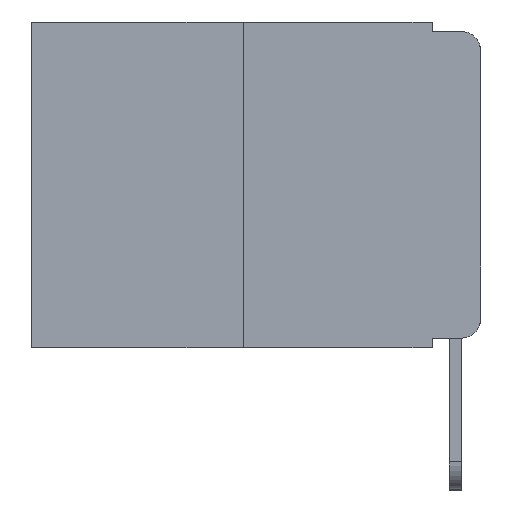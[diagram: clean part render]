
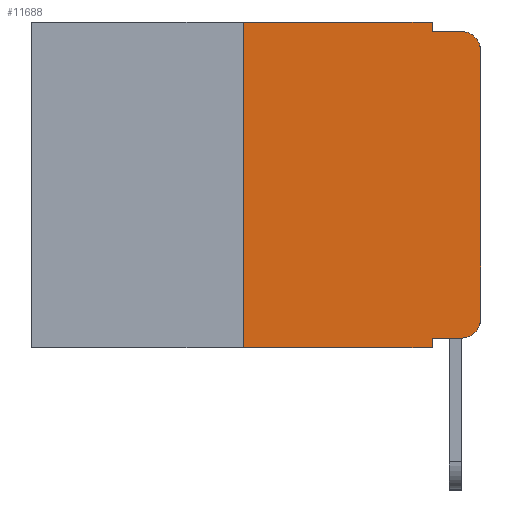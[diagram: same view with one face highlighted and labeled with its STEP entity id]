
A CAD part, left-side view. The second image highlights one B-rep face of the part: STEP entity #11688.
In plain terms, the highlighted planar face has unit normal (-1, 0, 0).
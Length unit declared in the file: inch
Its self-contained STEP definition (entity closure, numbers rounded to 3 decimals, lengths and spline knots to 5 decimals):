
#247 = DIRECTION ( 'NONE',  ( 0., 0., -1. ) ) ;
#393 = CARTESIAN_POINT ( 'NONE',  ( 0., 0.051, -0.333 ) ) ;
#453 = CARTESIAN_POINT ( 'NONE',  ( 0., 0., -0.313 ) ) ;
#469 = VECTOR ( 'NONE', #12345, 39.37008 ) ;
#862 = ORIENTED_EDGE ( 'NONE', *, *, #11897, .F. ) ;
#910 = DIRECTION ( 'NONE',  ( 0., -1., 0. ) ) ;
#989 = CARTESIAN_POINT ( 'NONE',  ( 0., 0.25, 0. ) ) ;
#1077 = DIRECTION ( 'NONE',  ( 0., 0., -1. ) ) ;
#1086 = EDGE_CURVE ( 'NONE', #10923, #11331, #10869, .T. ) ;
#1088 = DIRECTION ( 'NONE',  ( 0., -1., 0. ) ) ;
#1341 = EDGE_LOOP ( 'NONE', ( #8229, #8636, #10914, #2355, #1882, #6514, #6603, #862, #5809, #4588 ) ) ;
#1342 = DIRECTION ( 'NONE',  ( -1., 0., 0. ) ) ;
#1620 = VECTOR ( 'NONE', #12644, 39.37008 ) ;
#1882 = ORIENTED_EDGE ( 'NONE', *, *, #1086, .F. ) ;
#2343 = CARTESIAN_POINT ( 'NONE',  ( 0., 0.473, 0. ) ) ;
#2355 = ORIENTED_EDGE ( 'NONE', *, *, #12616, .F. ) ;
#2583 = VECTOR ( 'NONE', #9822, 39.37008 ) ;
#2612 = VERTEX_POINT ( 'NONE', #453 ) ;
#2708 = VERTEX_POINT ( 'NONE', #12746 ) ;
#2729 = VECTOR ( 'NONE', #10475, 39.37008 ) ;
#2891 = VECTOR ( 'NONE', #7727, 39.37008 ) ;
#2892 = CIRCLE ( 'NONE', #10574, 0.02 ) ;
#2956 = CARTESIAN_POINT ( 'NONE',  ( 0., 0., -0.03 ) ) ;
#3843 = CARTESIAN_POINT ( 'NONE',  ( 0., 0.051, 0. ) ) ;
#4492 = AXIS2_PLACEMENT_3D ( 'NONE', #7003, #6009, #12083 ) ;
#4588 = ORIENTED_EDGE ( 'NONE', *, *, #9158, .T. ) ;
#4644 = LINE ( 'NONE', #10712, #2891 ) ;
#4702 = LINE ( 'NONE', #7176, #11102 ) ;
#4929 = LINE ( 'NONE', #9195, #10697 ) ;
#5020 = CARTESIAN_POINT ( 'NONE',  ( 0., 0.051, -0.343 ) ) ;
#5229 = CARTESIAN_POINT ( 'NONE',  ( 0., 0., 0. ) ) ;
#5346 = CARTESIAN_POINT ( 'NONE',  ( 0., 0.25, 0. ) ) ;
#5636 = CARTESIAN_POINT ( 'NONE',  ( 0., 0.051, 0. ) ) ;
#5809 = ORIENTED_EDGE ( 'NONE', *, *, #6501, .T. ) ;
#6009 = DIRECTION ( 'NONE',  ( -1., 0., 0. ) ) ;
#6055 = LINE ( 'NONE', #393, #1620 ) ;
#6311 = CARTESIAN_POINT ( 'NONE',  ( 0., 0.051, -0.01 ) ) ;
#6501 = EDGE_CURVE ( 'NONE', #7918, #8531, #6055, .T. ) ;
#6514 = ORIENTED_EDGE ( 'NONE', *, *, #11779, .F. ) ;
#6603 = ORIENTED_EDGE ( 'NONE', *, *, #6868, .T. ) ;
#6658 = LINE ( 'NONE', #5636, #13190 ) ;
#6841 = EDGE_CURVE ( 'NONE', #10787, #2708, #12117, .T. ) ;
#6868 = EDGE_CURVE ( 'NONE', #13175, #12124, #4929, .T. ) ;
#7003 = CARTESIAN_POINT ( 'NONE',  ( 0., 0.02, -0.03 ) ) ;
#7176 = CARTESIAN_POINT ( 'NONE',  ( 0., 0.051, -0.01 ) ) ;
#7637 = VERTEX_POINT ( 'NONE', #6311 ) ;
#7662 = EDGE_CURVE ( 'NONE', #2612, #10787, #11311, .T. ) ;
#7727 = DIRECTION ( 'NONE',  ( 0., 0., -1. ) ) ;
#7918 = VERTEX_POINT ( 'NONE', #11704 ) ;
#8229 = ORIENTED_EDGE ( 'NONE', *, *, #7662, .T. ) ;
#8432 = CARTESIAN_POINT ( 'NONE',  ( 0., 0.02, -0.333 ) ) ;
#8531 = VERTEX_POINT ( 'NONE', #8432 ) ;
#8636 = ORIENTED_EDGE ( 'NONE', *, *, #6841, .T. ) ;
#9158 = EDGE_CURVE ( 'NONE', #8531, #2612, #2892, .T. ) ;
#9195 = CARTESIAN_POINT ( 'NONE',  ( 0., 0.473, -0.343 ) ) ;
#9479 = DIRECTION ( 'NONE',  ( 1., 0., 0. ) ) ;
#9592 = CARTESIAN_POINT ( 'NONE',  ( 0., 0.02, -0.313 ) ) ;
#9822 = DIRECTION ( 'NONE',  ( 0., 0., 1. ) ) ;
#10085 = AXIS2_PLACEMENT_3D ( 'NONE', #2343, #9479, #247 ) ;
#10475 = DIRECTION ( 'NONE',  ( 0., -1., 0. ) ) ;
#10574 = AXIS2_PLACEMENT_3D ( 'NONE', #9592, #1342, #12613 ) ;
#10608 = CARTESIAN_POINT ( 'NONE',  ( 0., 0.473, 0. ) ) ;
#10697 = VECTOR ( 'NONE', #910, 39.37008 ) ;
#10712 = CARTESIAN_POINT ( 'NONE',  ( 0., 0.051, 0. ) ) ;
#10787 = VERTEX_POINT ( 'NONE', #2956 ) ;
#10869 = LINE ( 'NONE', #10608, #2729 ) ;
#10914 = ORIENTED_EDGE ( 'NONE', *, *, #12159, .F. ) ;
#10923 = VERTEX_POINT ( 'NONE', #989 ) ;
#11102 = VECTOR ( 'NONE', #1088, 39.37008 ) ;
#11311 = LINE ( 'NONE', #5229, #469 ) ;
#11331 = VERTEX_POINT ( 'NONE', #3843 ) ;
#11688 = ADVANCED_FACE ( 'NONE', ( #12799 ), #12545, .F. ) ;
#11704 = CARTESIAN_POINT ( 'NONE',  ( 0., 0.051, -0.333 ) ) ;
#11779 = EDGE_CURVE ( 'NONE', #13175, #10923, #12951, .T. ) ;
#11897 = EDGE_CURVE ( 'NONE', #7918, #12124, #4644, .T. ) ;
#12083 = DIRECTION ( 'NONE',  ( 0., 0., -1. ) ) ;
#12117 = CIRCLE ( 'NONE', #4492, 0.02 ) ;
#12124 = VERTEX_POINT ( 'NONE', #5020 ) ;
#12159 = EDGE_CURVE ( 'NONE', #7637, #2708, #4702, .T. ) ;
#12345 = DIRECTION ( 'NONE',  ( 0., 0., 1. ) ) ;
#12545 = PLANE ( 'NONE',  #10085 ) ;
#12613 = DIRECTION ( 'NONE',  ( 0., 0., -1. ) ) ;
#12616 = EDGE_CURVE ( 'NONE', #11331, #7637, #6658, .T. ) ;
#12644 = DIRECTION ( 'NONE',  ( 0., -1., 0. ) ) ;
#12746 = CARTESIAN_POINT ( 'NONE',  ( 0., 0.02, -0.01 ) ) ;
#12799 = FACE_OUTER_BOUND ( 'NONE', #1341, .T. ) ;
#12951 = LINE ( 'NONE', #5346, #2583 ) ;
#12993 = CARTESIAN_POINT ( 'NONE',  ( 0., 0.25, -0.343 ) ) ;
#13175 = VERTEX_POINT ( 'NONE', #12993 ) ;
#13190 = VECTOR ( 'NONE', #1077, 39.37008 ) ;
